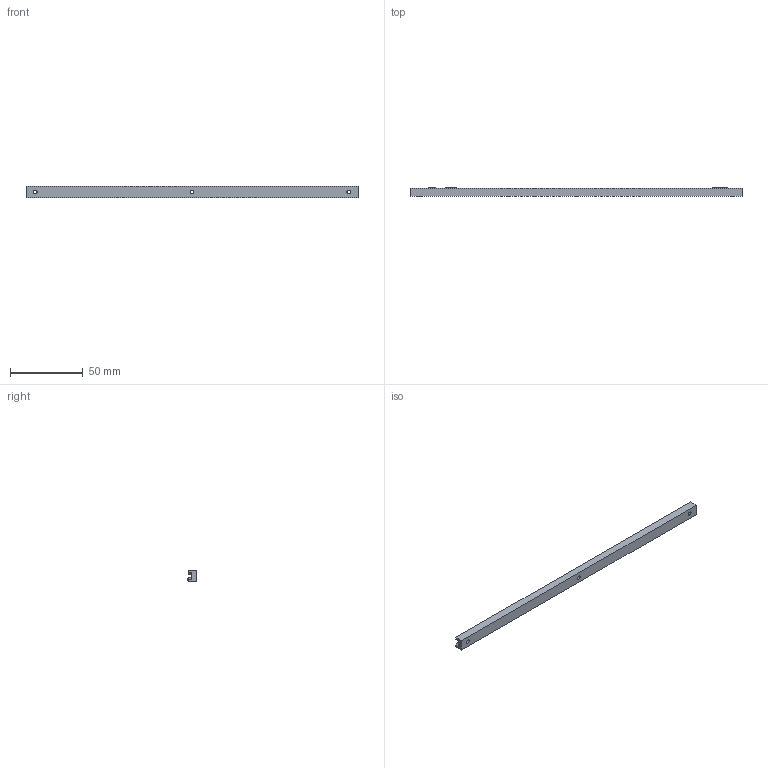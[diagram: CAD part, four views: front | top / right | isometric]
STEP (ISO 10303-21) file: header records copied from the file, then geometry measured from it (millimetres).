
FILE_DESCRIPTION (( 'STEP AP214' ), '1' );
FILE_NAME ('616-220-306.STEP', '2020-08-20T18:12:04', ( '' ), ( '' ), 'SwSTEP 2.0', 'SolidWorks 2020', '' );
FILE_SCHEMA (( 'AUTOMOTIVE_DESIGN' ));
Length unit declared in the file: inch
Products named in the file (1): 616-220-306
Bounding box: 228.6 x 5.66 x 7.92 mm (x, y, z)
Volume: 8887.9 mm3; surface area: 7403.4 mm2
Topology: 1 solids, 1 shells, 293 faces, 777 edges, 518 vertices
Faces by surface type: plane 178, bspline 103, cylinder 12
Entity records: 15193 total; most frequent: CARTESIAN_POINT 8524, ORIENTED_EDGE 1554, DIRECTION 989, EDGE_CURVE 777, LINE 535, VECTOR 535, VERTEX_POINT 518, EDGE_LOOP 331
